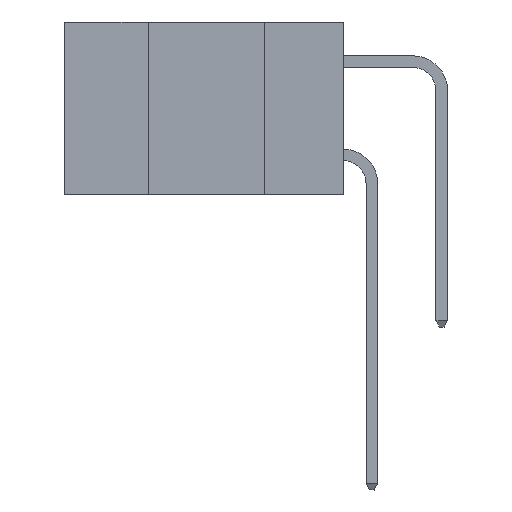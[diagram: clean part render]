
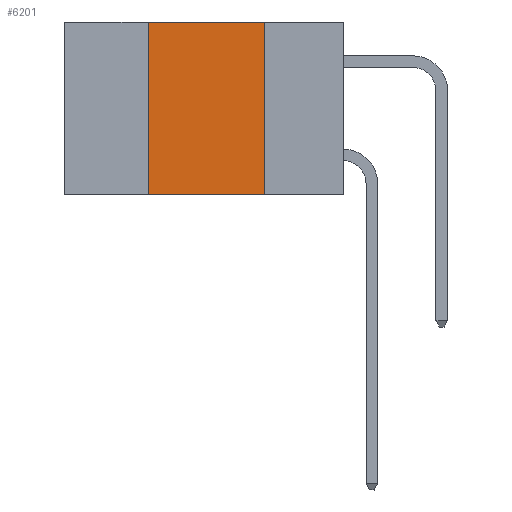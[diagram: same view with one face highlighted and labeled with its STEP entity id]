
A CAD part, left-side view. The second image highlights one B-rep face of the part: STEP entity #6201.
In plain terms, the highlighted planar face has unit normal (-1, 0, 0).
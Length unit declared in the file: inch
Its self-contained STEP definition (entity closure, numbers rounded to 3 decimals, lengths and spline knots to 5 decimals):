
#46 = DIRECTION ( 'NONE',  ( 0., -1., 0. ) ) ;
#467 = DIRECTION ( 'NONE',  ( 0., 0., -1. ) ) ;
#2019 = VERTEX_POINT ( 'NONE', #16956 ) ;
#2073 = VECTOR ( 'NONE', #3647, 39.37008 ) ;
#2447 = VECTOR ( 'NONE', #5608, 39.37008 ) ;
#2830 = VECTOR ( 'NONE', #467, 39.37008 ) ;
#3647 = DIRECTION ( 'NONE',  ( 0., 0., 1. ) ) ;
#3679 = LINE ( 'NONE', #7556, #17666 ) ;
#4156 = CARTESIAN_POINT ( 'NONE',  ( 0., 0.17, 0. ) ) ;
#5028 = VERTEX_POINT ( 'NONE', #9036 ) ;
#5608 = DIRECTION ( 'NONE',  ( 0., -1., 0. ) ) ;
#6201 = ADVANCED_FACE ( 'NONE', ( #19979 ), #11352, .F. ) ;
#6823 = ORIENTED_EDGE ( 'NONE', *, *, #8028, .F. ) ;
#7070 = VERTEX_POINT ( 'NONE', #15381 ) ;
#7213 = ORIENTED_EDGE ( 'NONE', *, *, #22965, .T. ) ;
#7556 = CARTESIAN_POINT ( 'NONE',  ( 0., 0.6, -0.37 ) ) ;
#8028 = EDGE_CURVE ( 'NONE', #5028, #2019, #22848, .T. ) ;
#8145 = ORIENTED_EDGE ( 'NONE', *, *, #9161, .F. ) ;
#8796 = LINE ( 'NONE', #18783, #2073 ) ;
#9036 = CARTESIAN_POINT ( 'NONE',  ( 0., 0.42, 0. ) ) ;
#9161 = EDGE_CURVE ( 'NONE', #2019, #7070, #12707, .T. ) ;
#11352 = PLANE ( 'NONE',  #23456 ) ;
#12707 = LINE ( 'NONE', #4156, #2830 ) ;
#12751 = EDGE_CURVE ( 'NONE', #13978, #5028, #8796, .T. ) ;
#13119 = CARTESIAN_POINT ( 'NONE',  ( 0., 0.6, 0. ) ) ;
#13271 = DIRECTION ( 'NONE',  ( 1., 0., 0. ) ) ;
#13978 = VERTEX_POINT ( 'NONE', #17534 ) ;
#15381 = CARTESIAN_POINT ( 'NONE',  ( 0., 0.17, -0.37 ) ) ;
#15430 = EDGE_LOOP ( 'NONE', ( #8145, #6823, #20980, #7213 ) ) ;
#16956 = CARTESIAN_POINT ( 'NONE',  ( 0., 0.17, 0. ) ) ;
#17534 = CARTESIAN_POINT ( 'NONE',  ( 0., 0.42, -0.37 ) ) ;
#17666 = VECTOR ( 'NONE', #46, 39.37008 ) ;
#18783 = CARTESIAN_POINT ( 'NONE',  ( 0., 0.42, 0. ) ) ;
#19979 = FACE_OUTER_BOUND ( 'NONE', #15430, .T. ) ;
#20712 = DIRECTION ( 'NONE',  ( 0., 0., -1. ) ) ;
#20980 = ORIENTED_EDGE ( 'NONE', *, *, #12751, .F. ) ;
#22848 = LINE ( 'NONE', #24025, #2447 ) ;
#22965 = EDGE_CURVE ( 'NONE', #13978, #7070, #3679, .T. ) ;
#23456 = AXIS2_PLACEMENT_3D ( 'NONE', #13119, #13271, #20712 ) ;
#24025 = CARTESIAN_POINT ( 'NONE',  ( 0., 0.6, 0. ) ) ;
